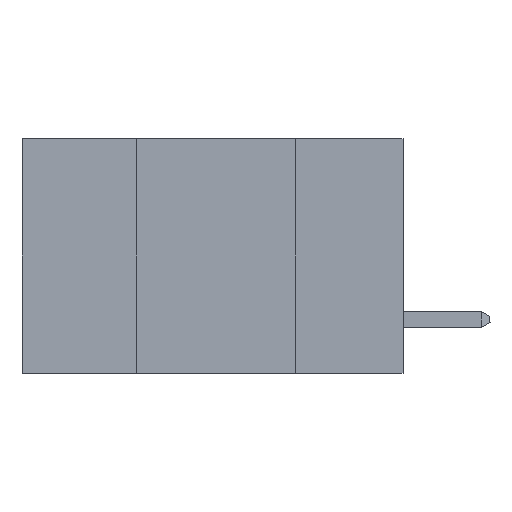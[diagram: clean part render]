
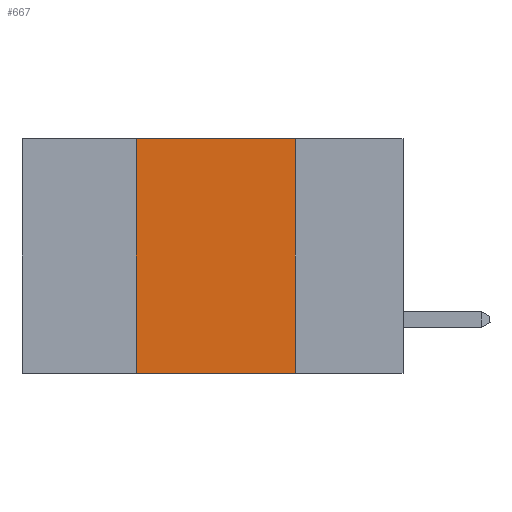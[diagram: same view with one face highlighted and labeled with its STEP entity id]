
A CAD part, left-side view. The second image highlights one B-rep face of the part: STEP entity #667.
In plain terms, the highlighted planar face has unit normal (-1, 0, 0).
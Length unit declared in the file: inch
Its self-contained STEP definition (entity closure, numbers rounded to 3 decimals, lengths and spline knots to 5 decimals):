
#277 = VECTOR ( 'NONE', #21609, 39.37008 ) ;
#667 = ADVANCED_FACE ( 'NONE', ( #3235 ), #33632, .F. ) ;
#1732 = DIRECTION ( 'NONE',  ( 0., 0., -1. ) ) ;
#2610 = DIRECTION ( 'NONE',  ( 0., -1., 0. ) ) ;
#3235 = FACE_OUTER_BOUND ( 'NONE', #7218, .T. ) ;
#4246 = VECTOR ( 'NONE', #38963, 39.37008 ) ;
#4533 = VECTOR ( 'NONE', #1732, 39.37008 ) ;
#4763 = ORIENTED_EDGE ( 'NONE', *, *, #38129, .F. ) ;
#7218 = EDGE_LOOP ( 'NONE', ( #4763, #19963, #45016, #17325 ) ) ;
#8508 = CARTESIAN_POINT ( 'NONE',  ( 0., 0.42, -0.37 ) ) ;
#8677 = CARTESIAN_POINT ( 'NONE',  ( 0., 0.6, -0.37 ) ) ;
#9619 = VECTOR ( 'NONE', #2610, 39.37008 ) ;
#10137 = CARTESIAN_POINT ( 'NONE',  ( 0., 0.42, 0. ) ) ;
#10473 = DIRECTION ( 'NONE',  ( 0., 0., -1. ) ) ;
#13264 = CARTESIAN_POINT ( 'NONE',  ( 0., 0.17, -0.37 ) ) ;
#14449 = CARTESIAN_POINT ( 'NONE',  ( 0., 0.6, 0. ) ) ;
#14766 = LINE ( 'NONE', #43514, #4533 ) ;
#17127 = VERTEX_POINT ( 'NONE', #13264 ) ;
#17325 = ORIENTED_EDGE ( 'NONE', *, *, #35297, .T. ) ;
#17965 = CARTESIAN_POINT ( 'NONE',  ( 0., 0.17, 0. ) ) ;
#19578 = VERTEX_POINT ( 'NONE', #8508 ) ;
#19963 = ORIENTED_EDGE ( 'NONE', *, *, #26495, .F. ) ;
#21609 = DIRECTION ( 'NONE',  ( 0., 0., 1. ) ) ;
#22240 = VERTEX_POINT ( 'NONE', #17965 ) ;
#23784 = LINE ( 'NONE', #8677, #4246 ) ;
#24647 = EDGE_CURVE ( 'NONE', #19578, #32097, #31108, .T. ) ;
#25258 = CARTESIAN_POINT ( 'NONE',  ( 0., 0.42, 0. ) ) ;
#26495 = EDGE_CURVE ( 'NONE', #32097, #22240, #38598, .T. ) ;
#31108 = LINE ( 'NONE', #25258, #277 ) ;
#32097 = VERTEX_POINT ( 'NONE', #10137 ) ;
#33632 = PLANE ( 'NONE',  #34364 ) ;
#34364 = AXIS2_PLACEMENT_3D ( 'NONE', #45022, #37270, #10473 ) ;
#35297 = EDGE_CURVE ( 'NONE', #19578, #17127, #23784, .T. ) ;
#37270 = DIRECTION ( 'NONE',  ( 1., 0., 0. ) ) ;
#38129 = EDGE_CURVE ( 'NONE', #22240, #17127, #14766, .T. ) ;
#38598 = LINE ( 'NONE', #14449, #9619 ) ;
#38963 = DIRECTION ( 'NONE',  ( 0., -1., 0. ) ) ;
#43514 = CARTESIAN_POINT ( 'NONE',  ( 0., 0.17, 0. ) ) ;
#45016 = ORIENTED_EDGE ( 'NONE', *, *, #24647, .F. ) ;
#45022 = CARTESIAN_POINT ( 'NONE',  ( 0., 0.6, 0. ) ) ;
